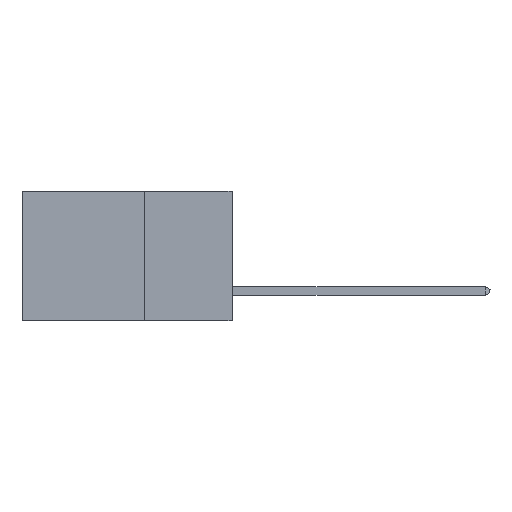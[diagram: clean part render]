
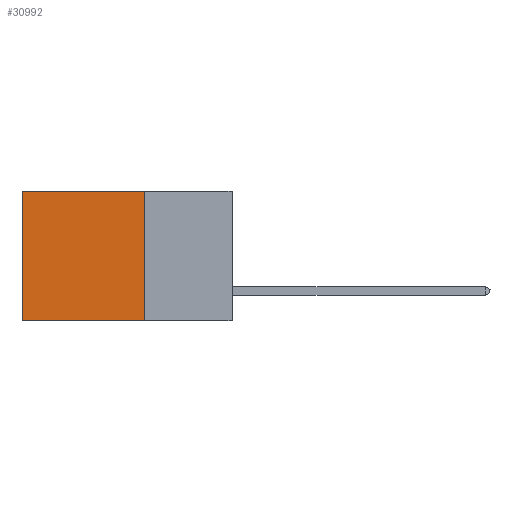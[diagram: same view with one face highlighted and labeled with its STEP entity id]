
A CAD part, left-side view. The second image highlights one B-rep face of the part: STEP entity #30992.
In plain terms, the highlighted planar face has unit normal (-1, 0, 0).
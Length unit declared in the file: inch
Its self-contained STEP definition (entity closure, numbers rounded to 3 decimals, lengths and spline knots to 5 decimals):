
#4404 = LINE ( 'NONE', #5983, #30797 ) ;
#4816 = LINE ( 'NONE', #27089, #7728 ) ;
#4872 = VERTEX_POINT ( 'NONE', #19198 ) ;
#5983 = CARTESIAN_POINT ( 'NONE',  ( 0.2875, 0.25, 0. ) ) ;
#7728 = VECTOR ( 'NONE', #32370, 39.37008 ) ;
#8708 = FACE_OUTER_BOUND ( 'NONE', #20402, .T. ) ;
#10840 = CARTESIAN_POINT ( 'NONE',  ( 0.2875, 0.25, -0.37 ) ) ;
#10965 = CARTESIAN_POINT ( 'NONE',  ( 0.2875, 0.25, 0. ) ) ;
#11273 = ORIENTED_EDGE ( 'NONE', *, *, #12390, .F. ) ;
#12390 = EDGE_CURVE ( 'NONE', #25385, #28829, #4404, .T. ) ;
#13283 = DIRECTION ( 'NONE',  ( 0., 1., 0. ) ) ;
#14207 = DIRECTION ( 'NONE',  ( 0., 0., -1. ) ) ;
#14323 = EDGE_CURVE ( 'NONE', #28829, #4872, #28404, .T. ) ;
#14987 = EDGE_CURVE ( 'NONE', #28143, #4872, #4816, .T. ) ;
#16301 = EDGE_CURVE ( 'NONE', #25385, #28143, #17511, .T. ) ;
#17302 = CARTESIAN_POINT ( 'NONE',  ( 0.2875, 0.25, 0. ) ) ;
#17396 = ORIENTED_EDGE ( 'NONE', *, *, #16301, .T. ) ;
#17511 = LINE ( 'NONE', #28297, #27451 ) ;
#18096 = DIRECTION ( 'NONE',  ( 0., 1., 0. ) ) ;
#19198 = CARTESIAN_POINT ( 'NONE',  ( 0.2875, 0.6, -0.37 ) ) ;
#20402 = EDGE_LOOP ( 'NONE', ( #30931, #23756, #11273, #17396 ) ) ;
#20699 = AXIS2_PLACEMENT_3D ( 'NONE', #10965, #26899, #14207 ) ;
#21332 = VECTOR ( 'NONE', #13283, 39.37008 ) ;
#22406 = CARTESIAN_POINT ( 'NONE',  ( 0.2875, 0.25, -0.37 ) ) ;
#22615 = CARTESIAN_POINT ( 'NONE',  ( 0.2875, 0.6, 0. ) ) ;
#23756 = ORIENTED_EDGE ( 'NONE', *, *, #14323, .F. ) ;
#24741 = PLANE ( 'NONE',  #20699 ) ;
#25385 = VERTEX_POINT ( 'NONE', #17302 ) ;
#26899 = DIRECTION ( 'NONE',  ( 1., 0., 0. ) ) ;
#27089 = CARTESIAN_POINT ( 'NONE',  ( 0.2875, 0.6, 0. ) ) ;
#27451 = VECTOR ( 'NONE', #18096, 39.37008 ) ;
#28143 = VERTEX_POINT ( 'NONE', #22615 ) ;
#28297 = CARTESIAN_POINT ( 'NONE',  ( 0.2875, 0.25, 0. ) ) ;
#28404 = LINE ( 'NONE', #10840, #21332 ) ;
#28829 = VERTEX_POINT ( 'NONE', #22406 ) ;
#30797 = VECTOR ( 'NONE', #32394, 39.37008 ) ;
#30931 = ORIENTED_EDGE ( 'NONE', *, *, #14987, .T. ) ;
#30992 = ADVANCED_FACE ( 'NONE', ( #8708 ), #24741, .F. ) ;
#32370 = DIRECTION ( 'NONE',  ( 0., 0., -1. ) ) ;
#32394 = DIRECTION ( 'NONE',  ( 0., 0., -1. ) ) ;
